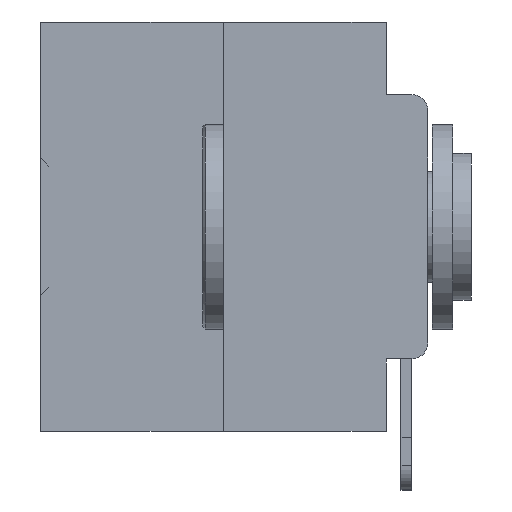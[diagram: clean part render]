
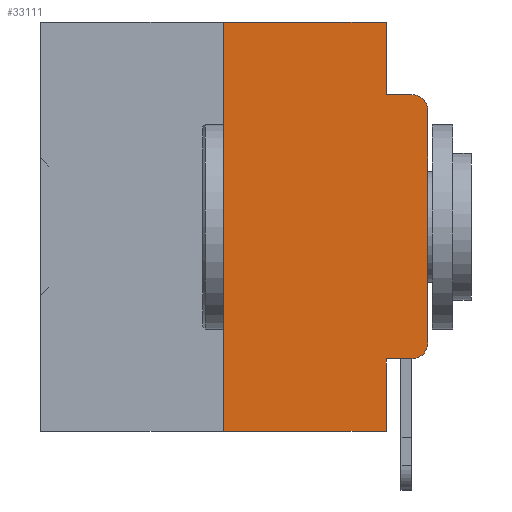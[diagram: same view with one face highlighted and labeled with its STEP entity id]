
A CAD part, left-side view. The second image highlights one B-rep face of the part: STEP entity #33111.
In plain terms, the highlighted planar face has unit normal (-1, 0, 0).
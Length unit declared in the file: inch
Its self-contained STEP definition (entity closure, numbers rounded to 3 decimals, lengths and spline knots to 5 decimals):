
#137 = CARTESIAN_POINT ( 'NONE',  ( 0., 0.473, 0. ) ) ;
#970 = LINE ( 'NONE', #12428, #32988 ) ;
#1495 = CARTESIAN_POINT ( 'NONE',  ( 0., 0.051, -0.4115 ) ) ;
#2484 = VECTOR ( 'NONE', #34830, 39.37008 ) ;
#3394 = VERTEX_POINT ( 'NONE', #31877 ) ;
#4151 = ORIENTED_EDGE ( 'NONE', *, *, #5405, .F. ) ;
#5405 = EDGE_CURVE ( 'NONE', #29555, #21220, #28684, .T. ) ;
#6254 = FACE_OUTER_BOUND ( 'NONE', #19404, .T. ) ;
#6951 = CARTESIAN_POINT ( 'NONE',  ( 0., 0.051, -0.4115 ) ) ;
#7410 = EDGE_CURVE ( 'NONE', #12054, #21220, #36992, .T. ) ;
#7601 = VERTEX_POINT ( 'NONE', #26948 ) ;
#7621 = AXIS2_PLACEMENT_3D ( 'NONE', #24642, #33191, #30495 ) ;
#8597 = LINE ( 'NONE', #23325, #23682 ) ;
#8652 = DIRECTION ( 'NONE',  ( 0., 0., -1. ) ) ;
#8960 = ORIENTED_EDGE ( 'NONE', *, *, #19618, .T. ) ;
#10535 = CARTESIAN_POINT ( 'NONE',  ( 0., 0.051, -0.5 ) ) ;
#11357 = DIRECTION ( 'NONE',  ( 0., 0., -1. ) ) ;
#11981 = VERTEX_POINT ( 'NONE', #28745 ) ;
#12054 = VERTEX_POINT ( 'NONE', #26174 ) ;
#12244 = AXIS2_PLACEMENT_3D ( 'NONE', #31700, #13952, #34581 ) ;
#12271 = EDGE_CURVE ( 'NONE', #3394, #32867, #970, .T. ) ;
#12428 = CARTESIAN_POINT ( 'NONE',  ( 0., 0.25, 0. ) ) ;
#12532 = VERTEX_POINT ( 'NONE', #1495 ) ;
#12544 = LINE ( 'NONE', #137, #28407 ) ;
#13002 = ORIENTED_EDGE ( 'NONE', *, *, #7410, .T. ) ;
#13952 = DIRECTION ( 'NONE',  ( -1., 0., 0. ) ) ;
#14359 = ORIENTED_EDGE ( 'NONE', *, *, #38524, .F. ) ;
#14784 = ORIENTED_EDGE ( 'NONE', *, *, #23145, .T. ) ;
#17036 = CARTESIAN_POINT ( 'NONE',  ( 0., 0., 0. ) ) ;
#17097 = DIRECTION ( 'NONE',  ( -1., 0., 0. ) ) ;
#17185 = ORIENTED_EDGE ( 'NONE', *, *, #22340, .F. ) ;
#17271 = CARTESIAN_POINT ( 'NONE',  ( 0., 0.473, -0.5 ) ) ;
#17680 = CARTESIAN_POINT ( 'NONE',  ( 0., 0.051, 0. ) ) ;
#19013 = DIRECTION ( 'NONE',  ( 0., -1., 0. ) ) ;
#19140 = VECTOR ( 'NONE', #19013, 39.37008 ) ;
#19404 = EDGE_LOOP ( 'NONE', ( #8960, #13002, #4151, #17185, #26568, #30538, #14784, #14359, #37976, #38226 ) ) ;
#19485 = LINE ( 'NONE', #17680, #25526 ) ;
#19618 = EDGE_CURVE ( 'NONE', #11981, #12054, #27595, .T. ) ;
#20226 = CARTESIAN_POINT ( 'NONE',  ( 0., 0.25, 0. ) ) ;
#20816 = VECTOR ( 'NONE', #36801, 39.37008 ) ;
#21220 = VERTEX_POINT ( 'NONE', #32752 ) ;
#21509 = DIRECTION ( 'NONE',  ( 0., -1., 0. ) ) ;
#22340 = EDGE_CURVE ( 'NONE', #7601, #29555, #8597, .T. ) ;
#23088 = EDGE_CURVE ( 'NONE', #36851, #11981, #35212, .T. ) ;
#23145 = EDGE_CURVE ( 'NONE', #3394, #32002, #25696, .T. ) ;
#23313 = CARTESIAN_POINT ( 'NONE',  ( 0., 0.02, -0.4115 ) ) ;
#23325 = CARTESIAN_POINT ( 'NONE',  ( 0., 0.051, 0. ) ) ;
#23682 = VECTOR ( 'NONE', #11357, 39.37008 ) ;
#24642 = CARTESIAN_POINT ( 'NONE',  ( 0., 0.473, 0. ) ) ;
#25526 = VECTOR ( 'NONE', #8652, 39.37008 ) ;
#25696 = LINE ( 'NONE', #17271, #2484 ) ;
#26174 = CARTESIAN_POINT ( 'NONE',  ( 0., 0., -0.1085 ) ) ;
#26568 = ORIENTED_EDGE ( 'NONE', *, *, #31073, .F. ) ;
#26948 = CARTESIAN_POINT ( 'NONE',  ( 0., 0.051, 0. ) ) ;
#27030 = LINE ( 'NONE', #6951, #19140 ) ;
#27585 = PLANE ( 'NONE',  #7621 ) ;
#27595 = LINE ( 'NONE', #17036, #35262 ) ;
#28407 = VECTOR ( 'NONE', #21509, 39.37008 ) ;
#28684 = LINE ( 'NONE', #33993, #20816 ) ;
#28745 = CARTESIAN_POINT ( 'NONE',  ( 0., 0., -0.3915 ) ) ;
#28925 = DIRECTION ( 'NONE',  ( 0., 0., 1. ) ) ;
#29555 = VERTEX_POINT ( 'NONE', #34245 ) ;
#30495 = DIRECTION ( 'NONE',  ( 0., 0., -1. ) ) ;
#30538 = ORIENTED_EDGE ( 'NONE', *, *, #12271, .F. ) ;
#31073 = EDGE_CURVE ( 'NONE', #32867, #7601, #12544, .T. ) ;
#31700 = CARTESIAN_POINT ( 'NONE',  ( 0., 0.02, -0.3915 ) ) ;
#31877 = CARTESIAN_POINT ( 'NONE',  ( 0., 0.25, -0.5 ) ) ;
#32002 = VERTEX_POINT ( 'NONE', #10535 ) ;
#32752 = CARTESIAN_POINT ( 'NONE',  ( 0., 0.02, -0.0885 ) ) ;
#32867 = VERTEX_POINT ( 'NONE', #20226 ) ;
#32988 = VECTOR ( 'NONE', #33177, 39.37008 ) ;
#33111 = ADVANCED_FACE ( 'NONE', ( #6254 ), #27585, .F. ) ;
#33177 = DIRECTION ( 'NONE',  ( 0., 0., 1. ) ) ;
#33191 = DIRECTION ( 'NONE',  ( 1., 0., 0. ) ) ;
#33993 = CARTESIAN_POINT ( 'NONE',  ( 0., 0.051, -0.0885 ) ) ;
#34245 = CARTESIAN_POINT ( 'NONE',  ( 0., 0.051, -0.0885 ) ) ;
#34581 = DIRECTION ( 'NONE',  ( 0., 0., -1. ) ) ;
#34658 = CARTESIAN_POINT ( 'NONE',  ( 0., 0.02, -0.1085 ) ) ;
#34830 = DIRECTION ( 'NONE',  ( 0., -1., 0. ) ) ;
#35212 = CIRCLE ( 'NONE', #12244, 0.02 ) ;
#35262 = VECTOR ( 'NONE', #28925, 39.37008 ) ;
#35393 = AXIS2_PLACEMENT_3D ( 'NONE', #34658, #17097, #37448 ) ;
#36654 = EDGE_CURVE ( 'NONE', #12532, #36851, #27030, .T. ) ;
#36801 = DIRECTION ( 'NONE',  ( 0., -1., 0. ) ) ;
#36851 = VERTEX_POINT ( 'NONE', #23313 ) ;
#36992 = CIRCLE ( 'NONE', #35393, 0.02 ) ;
#37448 = DIRECTION ( 'NONE',  ( 0., 0., -1. ) ) ;
#37976 = ORIENTED_EDGE ( 'NONE', *, *, #36654, .T. ) ;
#38226 = ORIENTED_EDGE ( 'NONE', *, *, #23088, .T. ) ;
#38524 = EDGE_CURVE ( 'NONE', #12532, #32002, #19485, .T. ) ;
